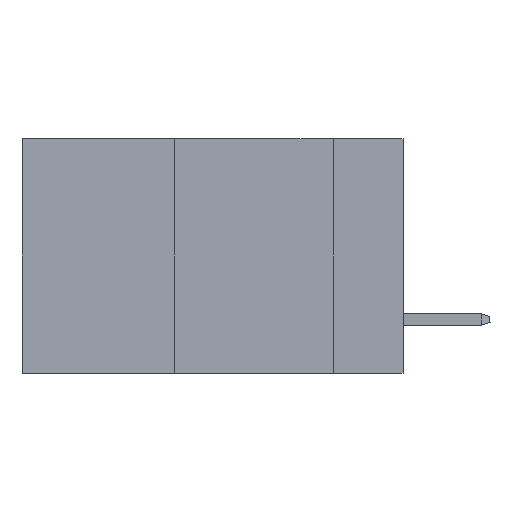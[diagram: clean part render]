
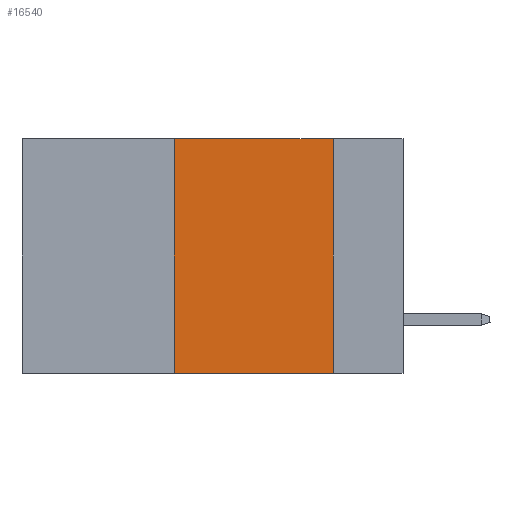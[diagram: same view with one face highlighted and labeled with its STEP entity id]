
A CAD part, left-side view. The second image highlights one B-rep face of the part: STEP entity #16540.
In plain terms, the highlighted planar face has unit normal (-1, 0, 0).
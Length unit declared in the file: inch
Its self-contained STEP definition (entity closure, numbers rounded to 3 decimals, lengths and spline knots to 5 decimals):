
#34 = ORIENTED_EDGE ( 'NONE', *, *, #16758, .F. ) ;
#450 = CARTESIAN_POINT ( 'NONE',  ( 0., 0.11, 0. ) ) ;
#479 = CARTESIAN_POINT ( 'NONE',  ( 0., 0.36, -0.37 ) ) ;
#584 = VECTOR ( 'NONE', #4583, 39.37008 ) ;
#658 = CARTESIAN_POINT ( 'NONE',  ( 0., 0.11, 0. ) ) ;
#1474 = VERTEX_POINT ( 'NONE', #479 ) ;
#1911 = DIRECTION ( 'NONE',  ( 0., -1., 0. ) ) ;
#2753 = VERTEX_POINT ( 'NONE', #5065 ) ;
#3447 = LINE ( 'NONE', #450, #14996 ) ;
#4156 = VERTEX_POINT ( 'NONE', #13218 ) ;
#4220 = CARTESIAN_POINT ( 'NONE',  ( 0., 0.6, 0. ) ) ;
#4320 = VERTEX_POINT ( 'NONE', #658 ) ;
#4334 = CARTESIAN_POINT ( 'NONE',  ( 0., 0.36, 0. ) ) ;
#4426 = LINE ( 'NONE', #4334, #584 ) ;
#4561 = ORIENTED_EDGE ( 'NONE', *, *, #14946, .T. ) ;
#4583 = DIRECTION ( 'NONE',  ( 0., 0., 1. ) ) ;
#5065 = CARTESIAN_POINT ( 'NONE',  ( 0., 0.11, -0.37 ) ) ;
#5112 = CARTESIAN_POINT ( 'NONE',  ( 0., 0.6, 0. ) ) ;
#6529 = LINE ( 'NONE', #5112, #17299 ) ;
#7350 = AXIS2_PLACEMENT_3D ( 'NONE', #4220, #10063, #12713 ) ;
#8096 = ORIENTED_EDGE ( 'NONE', *, *, #15119, .F. ) ;
#8747 = PLANE ( 'NONE',  #7350 ) ;
#8955 = LINE ( 'NONE', #14563, #12333 ) ;
#9208 = DIRECTION ( 'NONE',  ( 0., 0., -1. ) ) ;
#10063 = DIRECTION ( 'NONE',  ( 1., 0., 0. ) ) ;
#10155 = FACE_OUTER_BOUND ( 'NONE', #13605, .T. ) ;
#10792 = DIRECTION ( 'NONE',  ( 0., -1., 0. ) ) ;
#12333 = VECTOR ( 'NONE', #1911, 39.37008 ) ;
#12713 = DIRECTION ( 'NONE',  ( 0., 0., -1. ) ) ;
#13218 = CARTESIAN_POINT ( 'NONE',  ( 0., 0.36, 0. ) ) ;
#13605 = EDGE_LOOP ( 'NONE', ( #34, #8096, #17482, #4561 ) ) ;
#14563 = CARTESIAN_POINT ( 'NONE',  ( 0., 0.6, -0.37 ) ) ;
#14946 = EDGE_CURVE ( 'NONE', #1474, #2753, #8955, .T. ) ;
#14996 = VECTOR ( 'NONE', #9208, 39.37008 ) ;
#15119 = EDGE_CURVE ( 'NONE', #4156, #4320, #6529, .T. ) ;
#16180 = EDGE_CURVE ( 'NONE', #1474, #4156, #4426, .T. ) ;
#16540 = ADVANCED_FACE ( 'NONE', ( #10155 ), #8747, .F. ) ;
#16758 = EDGE_CURVE ( 'NONE', #4320, #2753, #3447, .T. ) ;
#17299 = VECTOR ( 'NONE', #10792, 39.37008 ) ;
#17482 = ORIENTED_EDGE ( 'NONE', *, *, #16180, .F. ) ;
